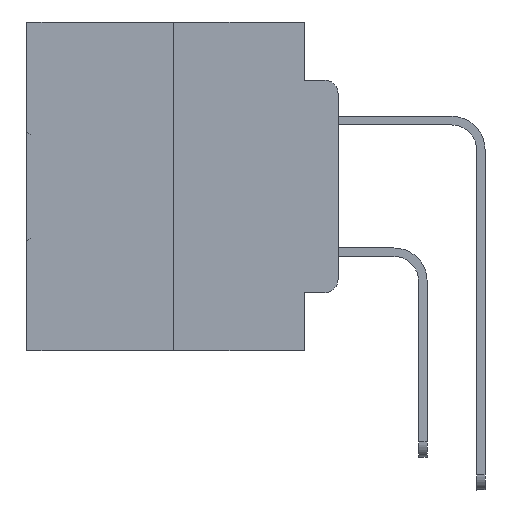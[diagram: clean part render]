
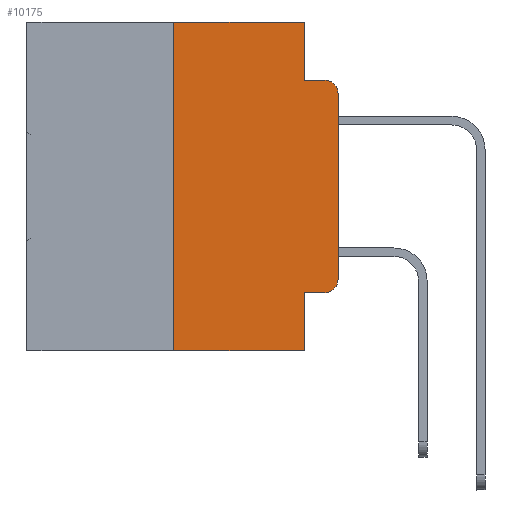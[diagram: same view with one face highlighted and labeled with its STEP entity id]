
A CAD part, left-side view. The second image highlights one B-rep face of the part: STEP entity #10175.
In plain terms, the highlighted planar face has unit normal (-1, 0, 0).
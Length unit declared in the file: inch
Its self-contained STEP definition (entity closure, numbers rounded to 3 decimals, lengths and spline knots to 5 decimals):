
#599 = AXIS2_PLACEMENT_3D ( 'NONE', #26420, #11567, #28912 ) ;
#628 = VERTEX_POINT ( 'NONE', #27222 ) ;
#671 = DIRECTION ( 'NONE',  ( 0., 0., 1. ) ) ;
#1257 = VERTEX_POINT ( 'NONE', #12909 ) ;
#1601 = EDGE_CURVE ( 'NONE', #24244, #9728, #2432, .T. ) ;
#2032 = EDGE_CURVE ( 'NONE', #24951, #1257, #28947, .T. ) ;
#2161 = CARTESIAN_POINT ( 'NONE',  ( 0., 0.051, -0.4115 ) ) ;
#2274 = VERTEX_POINT ( 'NONE', #2161 ) ;
#2432 = LINE ( 'NONE', #31032, #22351 ) ;
#2723 = AXIS2_PLACEMENT_3D ( 'NONE', #17818, #18032, #10289 ) ;
#2807 = CARTESIAN_POINT ( 'NONE',  ( 0., 0.02, -0.0885 ) ) ;
#5025 = EDGE_CURVE ( 'NONE', #26926, #9728, #25293, .T. ) ;
#6360 = LINE ( 'NONE', #19394, #25387 ) ;
#6726 = ORIENTED_EDGE ( 'NONE', *, *, #10763, .F. ) ;
#6745 = EDGE_CURVE ( 'NONE', #26278, #26926, #15102, .T. ) ;
#6852 = VERTEX_POINT ( 'NONE', #9906 ) ;
#7072 = DIRECTION ( 'NONE',  ( 0., 0., 1. ) ) ;
#7281 = DIRECTION ( 'NONE',  ( 0., -1., 0. ) ) ;
#8216 = LINE ( 'NONE', #25765, #14086 ) ;
#8419 = CARTESIAN_POINT ( 'NONE',  ( 0., 0.473, -0.5 ) ) ;
#9270 = VECTOR ( 'NONE', #17775, 39.37008 ) ;
#9728 = VERTEX_POINT ( 'NONE', #2807 ) ;
#9906 = CARTESIAN_POINT ( 'NONE',  ( 0., 0.25, 0. ) ) ;
#10175 = ADVANCED_FACE ( 'NONE', ( #29303 ), #22091, .F. ) ;
#10289 = DIRECTION ( 'NONE',  ( 0., 0., -1. ) ) ;
#10549 = VECTOR ( 'NONE', #16377, 39.37008 ) ;
#10763 = EDGE_CURVE ( 'NONE', #6852, #628, #6360, .T. ) ;
#10920 = DIRECTION ( 'NONE',  ( 0., 0., -1. ) ) ;
#11567 = DIRECTION ( 'NONE',  ( -1., 0., 0. ) ) ;
#12909 = CARTESIAN_POINT ( 'NONE',  ( 0., 0.051, -0.5 ) ) ;
#12986 = ORIENTED_EDGE ( 'NONE', *, *, #28989, .F. ) ;
#13037 = VECTOR ( 'NONE', #671, 39.37008 ) ;
#13712 = CARTESIAN_POINT ( 'NONE',  ( 0., 0.02, -0.4115 ) ) ;
#14086 = VECTOR ( 'NONE', #10920, 39.37008 ) ;
#14125 = CARTESIAN_POINT ( 'NONE',  ( 0., 0.051, -0.0885 ) ) ;
#14317 = VECTOR ( 'NONE', #7072, 39.37008 ) ;
#15102 = LINE ( 'NONE', #21917, #14317 ) ;
#15714 = ORIENTED_EDGE ( 'NONE', *, *, #2032, .T. ) ;
#16377 = DIRECTION ( 'NONE',  ( 0., 0., -1. ) ) ;
#17052 = ORIENTED_EDGE ( 'NONE', *, *, #5025, .T. ) ;
#17135 = CIRCLE ( 'NONE', #599, 0.02 ) ;
#17335 = AXIS2_PLACEMENT_3D ( 'NONE', #19642, #31891, #24604 ) ;
#17775 = DIRECTION ( 'NONE',  ( 0., -1., 0. ) ) ;
#17818 = CARTESIAN_POINT ( 'NONE',  ( 0., 0.02, -0.1085 ) ) ;
#18032 = DIRECTION ( 'NONE',  ( -1., 0., 0. ) ) ;
#18746 = ORIENTED_EDGE ( 'NONE', *, *, #30579, .F. ) ;
#18861 = LINE ( 'NONE', #28083, #13037 ) ;
#19394 = CARTESIAN_POINT ( 'NONE',  ( 0., 0.473, 0. ) ) ;
#19642 = CARTESIAN_POINT ( 'NONE',  ( 0., 0.473, 0. ) ) ;
#20546 = EDGE_LOOP ( 'NONE', ( #24654, #17052, #27115, #18746, #6726, #12986, #15714, #25837, #29351, #28602 ) ) ;
#20626 = EDGE_CURVE ( 'NONE', #29549, #26278, #17135, .T. ) ;
#21917 = CARTESIAN_POINT ( 'NONE',  ( 0., 0., 0. ) ) ;
#22091 = PLANE ( 'NONE',  #17335 ) ;
#22311 = EDGE_CURVE ( 'NONE', #2274, #29549, #29064, .T. ) ;
#22351 = VECTOR ( 'NONE', #30852, 39.37008 ) ;
#22916 = LINE ( 'NONE', #31143, #10549 ) ;
#23892 = VECTOR ( 'NONE', #7281, 39.37008 ) ;
#23936 = CARTESIAN_POINT ( 'NONE',  ( 0., 0.25, -0.5 ) ) ;
#24244 = VERTEX_POINT ( 'NONE', #14125 ) ;
#24604 = DIRECTION ( 'NONE',  ( 0., 0., -1. ) ) ;
#24629 = CARTESIAN_POINT ( 'NONE',  ( 0., 0., -0.1085 ) ) ;
#24654 = ORIENTED_EDGE ( 'NONE', *, *, #6745, .T. ) ;
#24951 = VERTEX_POINT ( 'NONE', #23936 ) ;
#25293 = CIRCLE ( 'NONE', #2723, 0.02 ) ;
#25387 = VECTOR ( 'NONE', #31757, 39.37008 ) ;
#25765 = CARTESIAN_POINT ( 'NONE',  ( 0., 0.051, 0. ) ) ;
#25837 = ORIENTED_EDGE ( 'NONE', *, *, #27324, .F. ) ;
#26278 = VERTEX_POINT ( 'NONE', #29067 ) ;
#26420 = CARTESIAN_POINT ( 'NONE',  ( 0., 0.02, -0.3915 ) ) ;
#26926 = VERTEX_POINT ( 'NONE', #24629 ) ;
#27115 = ORIENTED_EDGE ( 'NONE', *, *, #1601, .F. ) ;
#27222 = CARTESIAN_POINT ( 'NONE',  ( 0., 0.051, 0. ) ) ;
#27324 = EDGE_CURVE ( 'NONE', #2274, #1257, #22916, .T. ) ;
#27613 = CARTESIAN_POINT ( 'NONE',  ( 0., 0.051, -0.4115 ) ) ;
#28083 = CARTESIAN_POINT ( 'NONE',  ( 0., 0.25, 0. ) ) ;
#28602 = ORIENTED_EDGE ( 'NONE', *, *, #20626, .T. ) ;
#28912 = DIRECTION ( 'NONE',  ( 0., 0., -1. ) ) ;
#28947 = LINE ( 'NONE', #8419, #23892 ) ;
#28989 = EDGE_CURVE ( 'NONE', #24951, #6852, #18861, .T. ) ;
#29064 = LINE ( 'NONE', #27613, #9270 ) ;
#29067 = CARTESIAN_POINT ( 'NONE',  ( 0., 0., -0.3915 ) ) ;
#29303 = FACE_OUTER_BOUND ( 'NONE', #20546, .T. ) ;
#29351 = ORIENTED_EDGE ( 'NONE', *, *, #22311, .T. ) ;
#29549 = VERTEX_POINT ( 'NONE', #13712 ) ;
#30579 = EDGE_CURVE ( 'NONE', #628, #24244, #8216, .T. ) ;
#30852 = DIRECTION ( 'NONE',  ( 0., -1., 0. ) ) ;
#31032 = CARTESIAN_POINT ( 'NONE',  ( 0., 0.051, -0.0885 ) ) ;
#31143 = CARTESIAN_POINT ( 'NONE',  ( 0., 0.051, 0. ) ) ;
#31757 = DIRECTION ( 'NONE',  ( 0., -1., 0. ) ) ;
#31891 = DIRECTION ( 'NONE',  ( 1., 0., 0. ) ) ;
